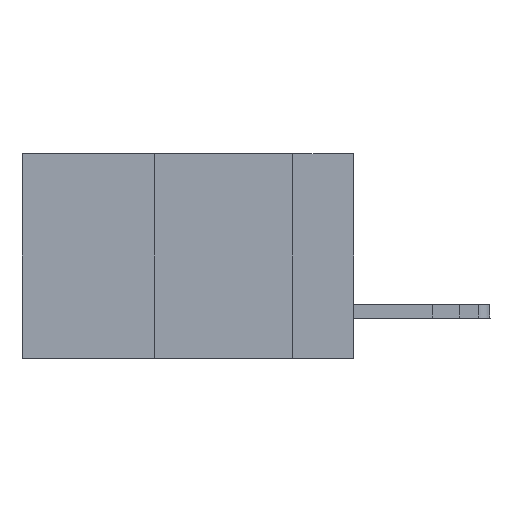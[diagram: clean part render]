
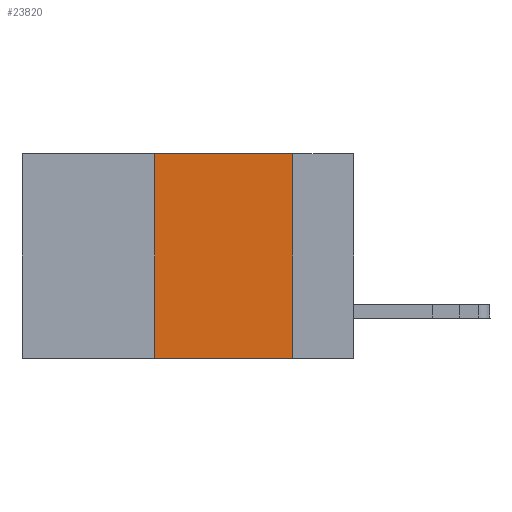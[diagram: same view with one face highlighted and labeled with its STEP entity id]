
A CAD part, left-side view. The second image highlights one B-rep face of the part: STEP entity #23820.
In plain terms, the highlighted planar face has unit normal (-1, 0, 0).
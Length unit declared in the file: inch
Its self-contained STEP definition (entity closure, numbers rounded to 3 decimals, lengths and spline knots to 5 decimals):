
#1529 = EDGE_CURVE ( 'NONE', #13848, #28093, #28629, .T. ) ;
#2124 = CARTESIAN_POINT ( 'NONE',  ( 0., 0.6, 0. ) ) ;
#2142 = VECTOR ( 'NONE', #15331, 39.37008 ) ;
#2616 = CARTESIAN_POINT ( 'NONE',  ( 0., 0.6, -0.37 ) ) ;
#2784 = EDGE_LOOP ( 'NONE', ( #11513, #35770, #29937, #7046 ) ) ;
#3664 = VECTOR ( 'NONE', #7976, 39.37008 ) ;
#6110 = DIRECTION ( 'NONE',  ( 1., 0., 0. ) ) ;
#7046 = ORIENTED_EDGE ( 'NONE', *, *, #15922, .T. ) ;
#7506 = DIRECTION ( 'NONE',  ( 0., -1., 0. ) ) ;
#7976 = DIRECTION ( 'NONE',  ( 0., 0., 1. ) ) ;
#8144 = DIRECTION ( 'NONE',  ( 0., -1., 0. ) ) ;
#8535 = LINE ( 'NONE', #2124, #34072 ) ;
#9168 = DIRECTION ( 'NONE',  ( 0., 0., -1. ) ) ;
#11513 = ORIENTED_EDGE ( 'NONE', *, *, #1529, .F. ) ;
#13848 = VERTEX_POINT ( 'NONE', #21913 ) ;
#14113 = CARTESIAN_POINT ( 'NONE',  ( 0., 0.36, 0. ) ) ;
#14623 = CARTESIAN_POINT ( 'NONE',  ( 0., 0.36, 0. ) ) ;
#15331 = DIRECTION ( 'NONE',  ( 0., 0., -1. ) ) ;
#15922 = EDGE_CURVE ( 'NONE', #24405, #28093, #32803, .T. ) ;
#16792 = VERTEX_POINT ( 'NONE', #14623 ) ;
#18170 = CARTESIAN_POINT ( 'NONE',  ( 0., 0.11, 0. ) ) ;
#21760 = EDGE_CURVE ( 'NONE', #24405, #16792, #33821, .T. ) ;
#21892 = VECTOR ( 'NONE', #8144, 39.37008 ) ;
#21913 = CARTESIAN_POINT ( 'NONE',  ( 0., 0.11, 0. ) ) ;
#23663 = FACE_OUTER_BOUND ( 'NONE', #2784, .T. ) ;
#23820 = ADVANCED_FACE ( 'NONE', ( #23663 ), #35330, .F. ) ;
#24405 = VERTEX_POINT ( 'NONE', #31684 ) ;
#26781 = CARTESIAN_POINT ( 'NONE',  ( 0., 0.6, 0. ) ) ;
#27466 = CARTESIAN_POINT ( 'NONE',  ( 0., 0.11, -0.37 ) ) ;
#28093 = VERTEX_POINT ( 'NONE', #27466 ) ;
#28629 = LINE ( 'NONE', #18170, #2142 ) ;
#28749 = EDGE_CURVE ( 'NONE', #16792, #13848, #8535, .T. ) ;
#29937 = ORIENTED_EDGE ( 'NONE', *, *, #21760, .F. ) ;
#31684 = CARTESIAN_POINT ( 'NONE',  ( 0., 0.36, -0.37 ) ) ;
#32803 = LINE ( 'NONE', #2616, #21892 ) ;
#33821 = LINE ( 'NONE', #14113, #3664 ) ;
#34072 = VECTOR ( 'NONE', #7506, 39.37008 ) ;
#35330 = PLANE ( 'NONE',  #37026 ) ;
#35770 = ORIENTED_EDGE ( 'NONE', *, *, #28749, .F. ) ;
#37026 = AXIS2_PLACEMENT_3D ( 'NONE', #26781, #6110, #9168 ) ;
